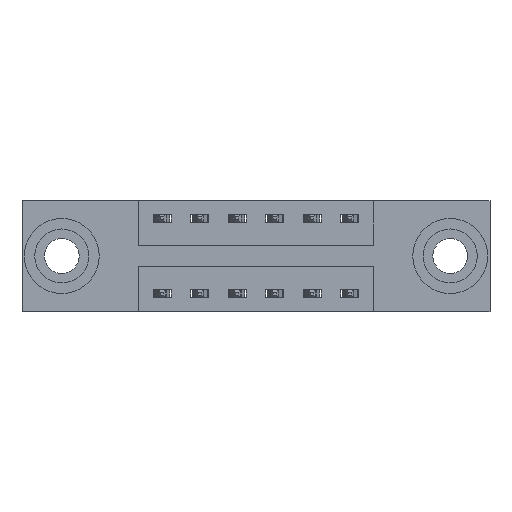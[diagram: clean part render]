
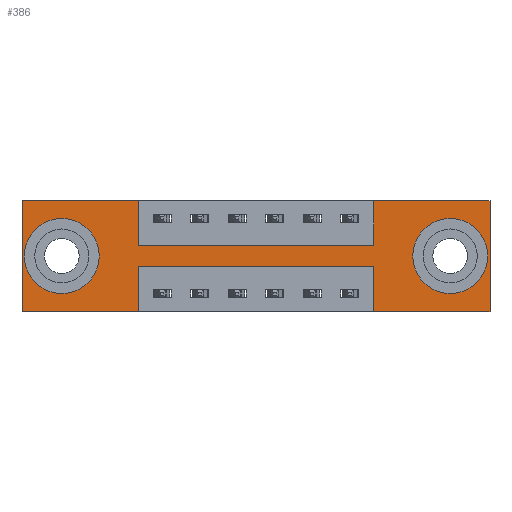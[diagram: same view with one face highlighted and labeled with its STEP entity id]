
A CAD part, front view. The second image highlights one B-rep face of the part: STEP entity #386.
In plain terms, the highlighted planar face has unit normal (0, -1, 0).
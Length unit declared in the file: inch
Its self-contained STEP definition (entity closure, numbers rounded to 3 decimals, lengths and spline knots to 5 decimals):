
#17 = DIRECTION ( 'NONE',  ( 0., 0., 1. ) ) ;
#203 = ORIENTED_EDGE ( 'NONE', *, *, #2359, .T. ) ;
#235 = ORIENTED_EDGE ( 'NONE', *, *, #4907, .F. ) ;
#364 = EDGE_CURVE ( 'NONE', #5245, #3110, #5934, .T. ) ;
#386 = ADVANCED_FACE ( 'NONE', ( #7580, #1866, #4273 ), #6536, .T. ) ;
#391 = CARTESIAN_POINT ( 'NONE',  ( 1.4275, 0., -0.107 ) ) ;
#426 = ORIENTED_EDGE ( 'NONE', *, *, #478, .T. ) ;
#429 = CARTESIAN_POINT ( 'NONE',  ( 0.1325, 0., -0.185 ) ) ;
#478 = EDGE_CURVE ( 'NONE', #2720, #6640, #8131, .T. ) ;
#647 = DIRECTION ( 'NONE',  ( 0., 0., -1. ) ) ;
#648 = CIRCLE ( 'NONE', #4151, 0.078 ) ;
#677 = AXIS2_PLACEMENT_3D ( 'NONE', #8417, #8340, #6308 ) ;
#761 = DIRECTION ( 'NONE',  ( 0., 1., 0. ) ) ;
#884 = CARTESIAN_POINT ( 'NONE',  ( 1.4275, 0., -0.185 ) ) ;
#982 = VERTEX_POINT ( 'NONE', #5726 ) ;
#1223 = EDGE_CURVE ( 'NONE', #982, #4099, #8545, .T. ) ;
#1249 = CARTESIAN_POINT ( 'NONE',  ( 0.3875, 0., -0.22 ) ) ;
#1315 = CARTESIAN_POINT ( 'NONE',  ( 0.1325, 0., -0.185 ) ) ;
#1371 = DIRECTION ( 'NONE',  ( 0., 0., -1. ) ) ;
#1386 = EDGE_CURVE ( 'NONE', #9014, #7188, #7035, .T. ) ;
#1609 = DIRECTION ( 'NONE',  ( -1., 0., 0. ) ) ;
#1666 = DIRECTION ( 'NONE',  ( 0., 1., 0. ) ) ;
#1805 = CARTESIAN_POINT ( 'NONE',  ( 0.3875, 0., 0. ) ) ;
#1816 = LINE ( 'NONE', #2503, #8924 ) ;
#1834 = CARTESIAN_POINT ( 'NONE',  ( 1.4275, 0., -0.185 ) ) ;
#1866 = FACE_BOUND ( 'NONE', #2440, .T. ) ;
#1893 = CARTESIAN_POINT ( 'NONE',  ( 0., 0., -0.37 ) ) ;
#2051 = EDGE_CURVE ( 'NONE', #5979, #7090, #5906, .T. ) ;
#2097 = VECTOR ( 'NONE', #7050, 39.37008 ) ;
#2100 = DIRECTION ( 'NONE',  ( 0., 0., 1. ) ) ;
#2150 = CARTESIAN_POINT ( 'NONE',  ( 0.3875, 0., 0. ) ) ;
#2255 = ORIENTED_EDGE ( 'NONE', *, *, #1386, .F. ) ;
#2359 = EDGE_CURVE ( 'NONE', #4601, #4080, #648, .T. ) ;
#2422 = CARTESIAN_POINT ( 'NONE',  ( 0.3875, 0., -0.22 ) ) ;
#2440 = EDGE_LOOP ( 'NONE', ( #7083, #426 ) ) ;
#2503 = CARTESIAN_POINT ( 'NONE',  ( 1.1725, 0., -0.37 ) ) ;
#2536 = EDGE_CURVE ( 'NONE', #4080, #4601, #5606, .T. ) ;
#2616 = CARTESIAN_POINT ( 'NONE',  ( 0., 0., 0. ) ) ;
#2720 = VERTEX_POINT ( 'NONE', #6081 ) ;
#2741 = AXIS2_PLACEMENT_3D ( 'NONE', #1315, #6410, #2100 ) ;
#2794 = LINE ( 'NONE', #3772, #8223 ) ;
#2848 = ORIENTED_EDGE ( 'NONE', *, *, #7478, .F. ) ;
#3092 = CARTESIAN_POINT ( 'NONE',  ( 1.4275, 0., -0.263 ) ) ;
#3110 = VERTEX_POINT ( 'NONE', #7128 ) ;
#3149 = VECTOR ( 'NONE', #6649, 39.37008 ) ;
#3328 = DIRECTION ( 'NONE',  ( 0., 0., 1. ) ) ;
#3423 = CARTESIAN_POINT ( 'NONE',  ( 1.56, 0., 0. ) ) ;
#3564 = CARTESIAN_POINT ( 'NONE',  ( 1.1725, 0., -0.22 ) ) ;
#3768 = DIRECTION ( 'NONE',  ( 0., 1., 0. ) ) ;
#3772 = CARTESIAN_POINT ( 'NONE',  ( 0.3875, 0., -0.37 ) ) ;
#3791 = VERTEX_POINT ( 'NONE', #1249 ) ;
#3810 = VERTEX_POINT ( 'NONE', #7084 ) ;
#3863 = EDGE_CURVE ( 'NONE', #3110, #982, #9078, .T. ) ;
#4010 = AXIS2_PLACEMENT_3D ( 'NONE', #884, #761, #647 ) ;
#4080 = VERTEX_POINT ( 'NONE', #3092 ) ;
#4099 = VERTEX_POINT ( 'NONE', #8731 ) ;
#4151 = AXIS2_PLACEMENT_3D ( 'NONE', #1834, #3768, #5414 ) ;
#4168 = EDGE_LOOP ( 'NONE', ( #235, #6829, #8648, #7897, #9329, #8762, #7485, #7552, #2848, #4351, #4260, #2255 ) ) ;
#4204 = CARTESIAN_POINT ( 'NONE',  ( 0.1325, 0., -0.107 ) ) ;
#4251 = LINE ( 'NONE', #2422, #5919 ) ;
#4260 = ORIENTED_EDGE ( 'NONE', *, *, #7913, .F. ) ;
#4273 = FACE_OUTER_BOUND ( 'NONE', #4168, .T. ) ;
#4351 = ORIENTED_EDGE ( 'NONE', *, *, #2051, .F. ) ;
#4471 = CARTESIAN_POINT ( 'NONE',  ( 1.1725, 0., -0.37 ) ) ;
#4489 = DIRECTION ( 'NONE',  ( 0., 0., -1. ) ) ;
#4601 = VERTEX_POINT ( 'NONE', #391 ) ;
#4645 = VECTOR ( 'NONE', #1371, 39.37008 ) ;
#4822 = CARTESIAN_POINT ( 'NONE',  ( 0.3875, 0., -0.37 ) ) ;
#4875 = DIRECTION ( 'NONE',  ( 0., 0., 1. ) ) ;
#4907 = EDGE_CURVE ( 'NONE', #3791, #9014, #2794, .T. ) ;
#4965 = CARTESIAN_POINT ( 'NONE',  ( 0., 0., 0. ) ) ;
#4981 = VECTOR ( 'NONE', #8206, 39.37008 ) ;
#4984 = EDGE_CURVE ( 'NONE', #9322, #3791, #4251, .T. ) ;
#5124 = VECTOR ( 'NONE', #1609, 39.37008 ) ;
#5245 = VERTEX_POINT ( 'NONE', #7669 ) ;
#5414 = DIRECTION ( 'NONE',  ( 0., 0., -1. ) ) ;
#5606 = CIRCLE ( 'NONE', #4010, 0.078 ) ;
#5638 = LINE ( 'NONE', #7811, #7323 ) ;
#5726 = CARTESIAN_POINT ( 'NONE',  ( 1.56, 0., 0. ) ) ;
#5739 = EDGE_LOOP ( 'NONE', ( #203, #7156 ) ) ;
#5760 = LINE ( 'NONE', #2616, #7616 ) ;
#5906 = LINE ( 'NONE', #9303, #6339 ) ;
#5919 = VECTOR ( 'NONE', #6653, 39.37008 ) ;
#5934 = LINE ( 'NONE', #6462, #2097 ) ;
#5979 = VERTEX_POINT ( 'NONE', #4965 ) ;
#6081 = CARTESIAN_POINT ( 'NONE',  ( 0.1325, 0., -0.263 ) ) ;
#6308 = DIRECTION ( 'NONE',  ( 0., 0., -1. ) ) ;
#6339 = VECTOR ( 'NONE', #9295, 39.37008 ) ;
#6410 = DIRECTION ( 'NONE',  ( 0., 1., 0. ) ) ;
#6462 = CARTESIAN_POINT ( 'NONE',  ( 1.1725, 0., 0. ) ) ;
#6532 = LINE ( 'NONE', #2150, #4645 ) ;
#6536 = PLANE ( 'NONE',  #677 ) ;
#6640 = VERTEX_POINT ( 'NONE', #4204 ) ;
#6649 = DIRECTION ( 'NONE',  ( 0., 0., -1. ) ) ;
#6653 = DIRECTION ( 'NONE',  ( -1., 0., 0. ) ) ;
#6829 = ORIENTED_EDGE ( 'NONE', *, *, #4984, .F. ) ;
#6837 = CARTESIAN_POINT ( 'NONE',  ( 0.3875, 0., -0.15 ) ) ;
#6866 = AXIS2_PLACEMENT_3D ( 'NONE', #429, #1666, #4875 ) ;
#7035 = LINE ( 'NONE', #1893, #5124 ) ;
#7047 = EDGE_CURVE ( 'NONE', #7666, #9322, #1816, .T. ) ;
#7050 = DIRECTION ( 'NONE',  ( 0., 0., 1. ) ) ;
#7083 = ORIENTED_EDGE ( 'NONE', *, *, #8214, .T. ) ;
#7084 = CARTESIAN_POINT ( 'NONE',  ( 0.3875, 0., -0.15 ) ) ;
#7090 = VERTEX_POINT ( 'NONE', #1805 ) ;
#7106 = LINE ( 'NONE', #6837, #4981 ) ;
#7110 = EDGE_CURVE ( 'NONE', #3810, #5245, #7106, .T. ) ;
#7115 = CARTESIAN_POINT ( 'NONE',  ( 0., 0., 0. ) ) ;
#7128 = CARTESIAN_POINT ( 'NONE',  ( 1.1725, 0., 0. ) ) ;
#7138 = DIRECTION ( 'NONE',  ( -1., 0., 0. ) ) ;
#7156 = ORIENTED_EDGE ( 'NONE', *, *, #2536, .T. ) ;
#7188 = VERTEX_POINT ( 'NONE', #8941 ) ;
#7282 = VECTOR ( 'NONE', #7783, 39.37008 ) ;
#7323 = VECTOR ( 'NONE', #7138, 39.37008 ) ;
#7478 = EDGE_CURVE ( 'NONE', #7090, #3810, #6532, .T. ) ;
#7485 = ORIENTED_EDGE ( 'NONE', *, *, #364, .F. ) ;
#7518 = CIRCLE ( 'NONE', #2741, 0.078 ) ;
#7552 = ORIENTED_EDGE ( 'NONE', *, *, #7110, .F. ) ;
#7580 = FACE_BOUND ( 'NONE', #5739, .T. ) ;
#7616 = VECTOR ( 'NONE', #3328, 39.37008 ) ;
#7666 = VERTEX_POINT ( 'NONE', #4471 ) ;
#7669 = CARTESIAN_POINT ( 'NONE',  ( 1.1725, 0., -0.15 ) ) ;
#7783 = DIRECTION ( 'NONE',  ( 1., 0., 0. ) ) ;
#7811 = CARTESIAN_POINT ( 'NONE',  ( 0., 0., -0.37 ) ) ;
#7897 = ORIENTED_EDGE ( 'NONE', *, *, #8231, .F. ) ;
#7913 = EDGE_CURVE ( 'NONE', #7188, #5979, #5760, .T. ) ;
#8131 = CIRCLE ( 'NONE', #6866, 0.078 ) ;
#8206 = DIRECTION ( 'NONE',  ( 1., 0., 0. ) ) ;
#8214 = EDGE_CURVE ( 'NONE', #6640, #2720, #7518, .T. ) ;
#8223 = VECTOR ( 'NONE', #4489, 39.37008 ) ;
#8231 = EDGE_CURVE ( 'NONE', #4099, #7666, #5638, .T. ) ;
#8340 = DIRECTION ( 'NONE',  ( 0., -1., 0. ) ) ;
#8417 = CARTESIAN_POINT ( 'NONE',  ( 0., 0., -0.37 ) ) ;
#8545 = LINE ( 'NONE', #3423, #3149 ) ;
#8648 = ORIENTED_EDGE ( 'NONE', *, *, #7047, .F. ) ;
#8731 = CARTESIAN_POINT ( 'NONE',  ( 1.56, 0., -0.37 ) ) ;
#8762 = ORIENTED_EDGE ( 'NONE', *, *, #3863, .F. ) ;
#8924 = VECTOR ( 'NONE', #17, 39.37008 ) ;
#8941 = CARTESIAN_POINT ( 'NONE',  ( 0., 0., -0.37 ) ) ;
#9014 = VERTEX_POINT ( 'NONE', #4822 ) ;
#9078 = LINE ( 'NONE', #7115, #7282 ) ;
#9295 = DIRECTION ( 'NONE',  ( 1., 0., 0. ) ) ;
#9303 = CARTESIAN_POINT ( 'NONE',  ( 0., 0., 0. ) ) ;
#9322 = VERTEX_POINT ( 'NONE', #3564 ) ;
#9329 = ORIENTED_EDGE ( 'NONE', *, *, #1223, .F. ) ;
